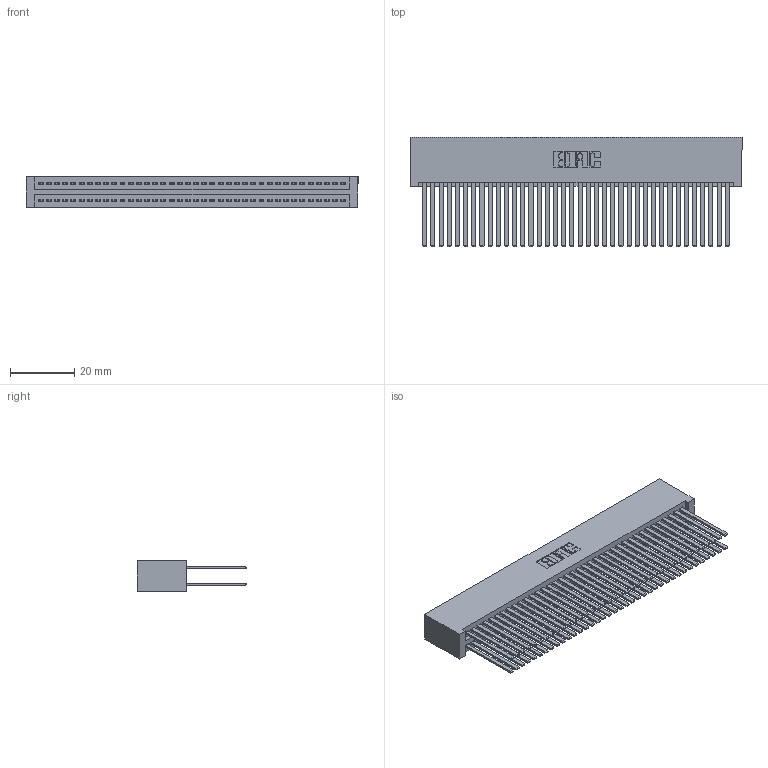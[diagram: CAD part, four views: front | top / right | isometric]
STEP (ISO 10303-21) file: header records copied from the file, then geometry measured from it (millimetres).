
FILE_DESCRIPTION (( 'STEP AP203' ), '1' );
FILE_NAME ('345-076-544-201.STEP', '2019-10-31T13:02:28', ( '' ), ( '' ), 'SwSTEP 2.0', 'SolidWorks 2016', '' );
FILE_SCHEMA (( 'CONFIG_CONTROL_DESIGN' ));
Length unit declared in the file: inch
Products named in the file (3): 345 Part_No Mounting Lugs; 345-076-544-201; 345-292-001_345-293-144
Assembly tree (77 placements, depth 2):
  345-076-544-201
    345 Part_No Mounting Lugs
    345-292-001_345-293-144  x76
Bounding box: 103.12 x 33.96 x 9.4 mm (x, y, z)
Volume: 11661.7 mm3; surface area: 20586.3 mm2
Topology: 77 solids, 77 shells, 3462 faces, 10273 edges, 6746 vertices
Faces by surface type: plane 2280, cylinder 1182
Entity records: 29893 total; most frequent: CARTESIAN_POINT 5012, ORIENTED_EDGE 4946, DIRECTION 4417, EDGE_CURVE 2473, LINE 2201, VECTOR 2201, VERTEX_POINT 1646, AXIS2_PLACEMENT_3D 1108
